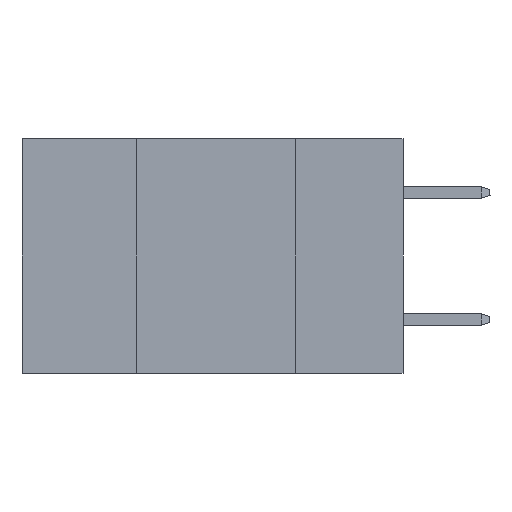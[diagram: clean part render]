
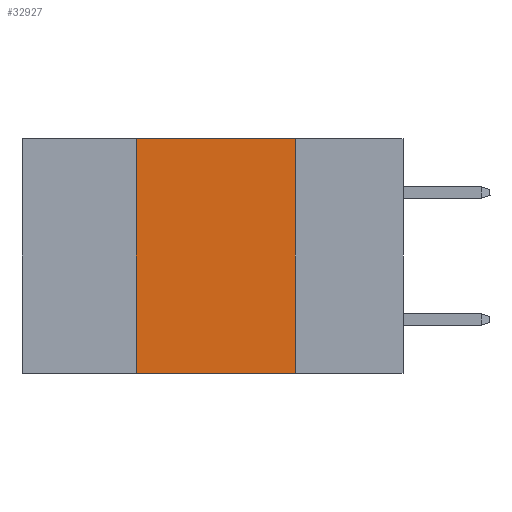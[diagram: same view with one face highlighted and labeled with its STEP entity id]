
A CAD part, left-side view. The second image highlights one B-rep face of the part: STEP entity #32927.
In plain terms, the highlighted planar face has unit normal (-1, 0, 0).
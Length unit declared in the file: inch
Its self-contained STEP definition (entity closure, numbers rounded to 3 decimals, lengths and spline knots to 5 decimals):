
#2506 = DIRECTION ( 'NONE',  ( 0., 0., -1. ) ) ;
#3195 = CARTESIAN_POINT ( 'NONE',  ( 0., 0.42, 0. ) ) ;
#3596 = DIRECTION ( 'NONE',  ( 0., -1., 0. ) ) ;
#4114 = VECTOR ( 'NONE', #2506, 39.37008 ) ;
#4255 = CARTESIAN_POINT ( 'NONE',  ( 0., 0.42, -0.37 ) ) ;
#10935 = EDGE_LOOP ( 'NONE', ( #41309, #13400, #33763, #42578 ) ) ;
#11116 = EDGE_CURVE ( 'NONE', #30910, #28198, #24035, .T. ) ;
#13400 = ORIENTED_EDGE ( 'NONE', *, *, #23968, .F. ) ;
#13440 = LINE ( 'NONE', #44123, #4114 ) ;
#16711 = PLANE ( 'NONE',  #25044 ) ;
#18567 = CARTESIAN_POINT ( 'NONE',  ( 0., 0.17, -0.37 ) ) ;
#20958 = CARTESIAN_POINT ( 'NONE',  ( 0., 0.6, 0. ) ) ;
#21183 = LINE ( 'NONE', #20958, #40560 ) ;
#21630 = DIRECTION ( 'NONE',  ( 0., -1., 0. ) ) ;
#22638 = EDGE_CURVE ( 'NONE', #30910, #30300, #34505, .T. ) ;
#23326 = CARTESIAN_POINT ( 'NONE',  ( 0., 0.6, 0. ) ) ;
#23968 = EDGE_CURVE ( 'NONE', #30300, #32347, #21183, .T. ) ;
#24035 = LINE ( 'NONE', #34472, #32450 ) ;
#25044 = AXIS2_PLACEMENT_3D ( 'NONE', #23326, #37185, #41018 ) ;
#27706 = DIRECTION ( 'NONE',  ( 0., 0., 1. ) ) ;
#28198 = VERTEX_POINT ( 'NONE', #18567 ) ;
#30300 = VERTEX_POINT ( 'NONE', #3195 ) ;
#30591 = FACE_OUTER_BOUND ( 'NONE', #10935, .T. ) ;
#30910 = VERTEX_POINT ( 'NONE', #4255 ) ;
#32347 = VERTEX_POINT ( 'NONE', #42909 ) ;
#32450 = VECTOR ( 'NONE', #3596, 39.37008 ) ;
#32927 = ADVANCED_FACE ( 'NONE', ( #30591 ), #16711, .F. ) ;
#33763 = ORIENTED_EDGE ( 'NONE', *, *, #22638, .F. ) ;
#34472 = CARTESIAN_POINT ( 'NONE',  ( 0., 0.6, -0.37 ) ) ;
#34505 = LINE ( 'NONE', #34738, #38321 ) ;
#34738 = CARTESIAN_POINT ( 'NONE',  ( 0., 0.42, 0. ) ) ;
#35947 = EDGE_CURVE ( 'NONE', #32347, #28198, #13440, .T. ) ;
#37185 = DIRECTION ( 'NONE',  ( 1., 0., 0. ) ) ;
#38321 = VECTOR ( 'NONE', #27706, 39.37008 ) ;
#40560 = VECTOR ( 'NONE', #21630, 39.37008 ) ;
#41018 = DIRECTION ( 'NONE',  ( 0., 0., -1. ) ) ;
#41309 = ORIENTED_EDGE ( 'NONE', *, *, #35947, .F. ) ;
#42578 = ORIENTED_EDGE ( 'NONE', *, *, #11116, .T. ) ;
#42909 = CARTESIAN_POINT ( 'NONE',  ( 0., 0.17, 0. ) ) ;
#44123 = CARTESIAN_POINT ( 'NONE',  ( 0., 0.17, 0. ) ) ;
